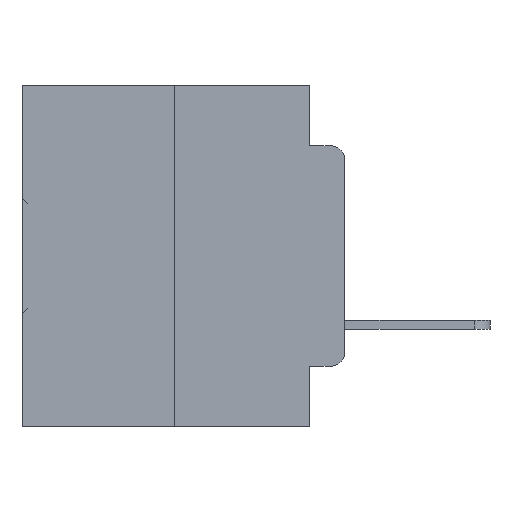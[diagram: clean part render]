
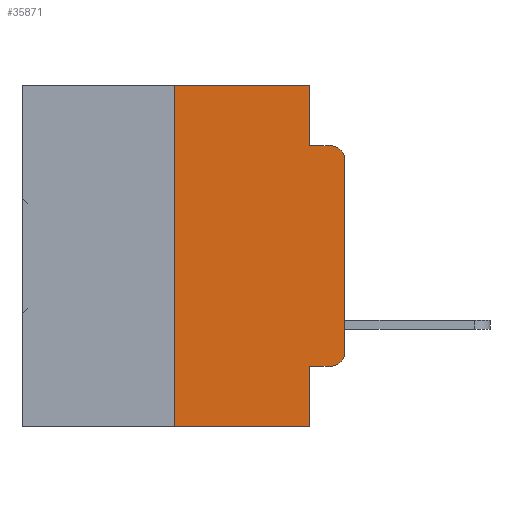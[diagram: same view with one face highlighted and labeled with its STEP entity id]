
A CAD part, left-side view. The second image highlights one B-rep face of the part: STEP entity #35871.
In plain terms, the highlighted planar face has unit normal (-1, 0, 0).
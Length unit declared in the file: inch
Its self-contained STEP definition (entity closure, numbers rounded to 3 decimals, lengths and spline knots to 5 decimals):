
#380 = EDGE_CURVE ( 'NONE', #27012, #5981, #12799, .T. ) ;
#2295 = EDGE_CURVE ( 'NONE', #11353, #27012, #8159, .T. ) ;
#2344 = EDGE_CURVE ( 'NONE', #18755, #28201, #34345, .T. ) ;
#4235 = EDGE_CURVE ( 'NONE', #11353, #32620, #6273, .T. ) ;
#4344 = VERTEX_POINT ( 'NONE', #6306 ) ;
#4665 = VECTOR ( 'NONE', #10213, 39.37008 ) ;
#4811 = VERTEX_POINT ( 'NONE', #8684 ) ;
#4935 = ORIENTED_EDGE ( 'NONE', *, *, #17738, .F. ) ;
#5347 = DIRECTION ( 'NONE',  ( 0., 0., 1. ) ) ;
#5734 = VERTEX_POINT ( 'NONE', #20676 ) ;
#5981 = VERTEX_POINT ( 'NONE', #10406 ) ;
#6125 = DIRECTION ( 'NONE',  ( 0., 0., -1. ) ) ;
#6170 = EDGE_CURVE ( 'NONE', #5734, #18755, #30769, .T. ) ;
#6264 = CARTESIAN_POINT ( 'NONE',  ( 0., 0.051, -0.5 ) ) ;
#6273 = LINE ( 'NONE', #8712, #20634 ) ;
#6306 = CARTESIAN_POINT ( 'NONE',  ( 0., 0.051, -0.0885 ) ) ;
#6311 = EDGE_LOOP ( 'NONE', ( #21344, #27413, #25255, #4935, #19779, #27445, #12371, #16758, #21984, #7515 ) ) ;
#7210 = DIRECTION ( 'NONE',  ( -1., 0., 0. ) ) ;
#7326 = CARTESIAN_POINT ( 'NONE',  ( 0., 0.051, -0.0885 ) ) ;
#7515 = ORIENTED_EDGE ( 'NONE', *, *, #380, .T. ) ;
#8159 = LINE ( 'NONE', #27965, #13971 ) ;
#8195 = LINE ( 'NONE', #25158, #14007 ) ;
#8247 = CARTESIAN_POINT ( 'NONE',  ( 0., 0.25, 0. ) ) ;
#8450 = AXIS2_PLACEMENT_3D ( 'NONE', #24183, #7210, #26970 ) ;
#8602 = PLANE ( 'NONE',  #15522 ) ;
#8684 = CARTESIAN_POINT ( 'NONE',  ( 0., 0.02, -0.0885 ) ) ;
#8712 = CARTESIAN_POINT ( 'NONE',  ( 0., 0.051, 0. ) ) ;
#10178 = CARTESIAN_POINT ( 'NONE',  ( 0., 0.051, -0.4115 ) ) ;
#10213 = DIRECTION ( 'NONE',  ( 0., -1., 0. ) ) ;
#10406 = CARTESIAN_POINT ( 'NONE',  ( 0., 0., -0.3915 ) ) ;
#10719 = CARTESIAN_POINT ( 'NONE',  ( 0., 0.473, -0.5 ) ) ;
#11011 = CARTESIAN_POINT ( 'NONE',  ( 0., 0.051, 0. ) ) ;
#11353 = VERTEX_POINT ( 'NONE', #10178 ) ;
#11428 = LINE ( 'NONE', #11011, #25590 ) ;
#12371 = ORIENTED_EDGE ( 'NONE', *, *, #26844, .T. ) ;
#12799 = CIRCLE ( 'NONE', #13096, 0.02 ) ;
#13096 = AXIS2_PLACEMENT_3D ( 'NONE', #14127, #33549, #17056 ) ;
#13809 = DIRECTION ( 'NONE',  ( 0., 0., 1. ) ) ;
#13971 = VECTOR ( 'NONE', #28083, 39.37008 ) ;
#14007 = VECTOR ( 'NONE', #13809, 39.37008 ) ;
#14127 = CARTESIAN_POINT ( 'NONE',  ( 0., 0.02, -0.3915 ) ) ;
#15522 = AXIS2_PLACEMENT_3D ( 'NONE', #33758, #17275, #6125 ) ;
#15587 = VERTEX_POINT ( 'NONE', #25623 ) ;
#16025 = VECTOR ( 'NONE', #5347, 39.37008 ) ;
#16758 = ORIENTED_EDGE ( 'NONE', *, *, #4235, .F. ) ;
#17056 = DIRECTION ( 'NONE',  ( 0., 0., -1. ) ) ;
#17275 = DIRECTION ( 'NONE',  ( 1., 0., 0. ) ) ;
#17738 = EDGE_CURVE ( 'NONE', #28201, #4344, #11428, .T. ) ;
#18173 = CIRCLE ( 'NONE', #8450, 0.02 ) ;
#18755 = VERTEX_POINT ( 'NONE', #28562 ) ;
#19598 = VECTOR ( 'NONE', #30289, 39.37008 ) ;
#19684 = EDGE_CURVE ( 'NONE', #4344, #4811, #19969, .T. ) ;
#19779 = ORIENTED_EDGE ( 'NONE', *, *, #2344, .F. ) ;
#19847 = VECTOR ( 'NONE', #26051, 39.37008 ) ;
#19969 = LINE ( 'NONE', #7326, #4665 ) ;
#20634 = VECTOR ( 'NONE', #28409, 39.37008 ) ;
#20676 = CARTESIAN_POINT ( 'NONE',  ( 0., 0.25, -0.5 ) ) ;
#21344 = ORIENTED_EDGE ( 'NONE', *, *, #30696, .T. ) ;
#21545 = EDGE_CURVE ( 'NONE', #15587, #4811, #18173, .T. ) ;
#21984 = ORIENTED_EDGE ( 'NONE', *, *, #2295, .T. ) ;
#24183 = CARTESIAN_POINT ( 'NONE',  ( 0., 0.02, -0.1085 ) ) ;
#25158 = CARTESIAN_POINT ( 'NONE',  ( 0., 0., 0. ) ) ;
#25255 = ORIENTED_EDGE ( 'NONE', *, *, #19684, .F. ) ;
#25590 = VECTOR ( 'NONE', #33322, 39.37008 ) ;
#25623 = CARTESIAN_POINT ( 'NONE',  ( 0., 0., -0.1085 ) ) ;
#26051 = DIRECTION ( 'NONE',  ( 0., -1., 0. ) ) ;
#26173 = CARTESIAN_POINT ( 'NONE',  ( 0., 0.051, 0. ) ) ;
#26844 = EDGE_CURVE ( 'NONE', #5734, #32620, #34123, .T. ) ;
#26970 = DIRECTION ( 'NONE',  ( 0., 0., -1. ) ) ;
#27012 = VERTEX_POINT ( 'NONE', #34202 ) ;
#27413 = ORIENTED_EDGE ( 'NONE', *, *, #21545, .T. ) ;
#27445 = ORIENTED_EDGE ( 'NONE', *, *, #6170, .F. ) ;
#27965 = CARTESIAN_POINT ( 'NONE',  ( 0., 0.051, -0.4115 ) ) ;
#28083 = DIRECTION ( 'NONE',  ( 0., -1., 0. ) ) ;
#28201 = VERTEX_POINT ( 'NONE', #26173 ) ;
#28409 = DIRECTION ( 'NONE',  ( 0., 0., -1. ) ) ;
#28562 = CARTESIAN_POINT ( 'NONE',  ( 0., 0.25, 0. ) ) ;
#28573 = FACE_OUTER_BOUND ( 'NONE', #6311, .T. ) ;
#28670 = CARTESIAN_POINT ( 'NONE',  ( 0., 0.473, 0. ) ) ;
#30289 = DIRECTION ( 'NONE',  ( 0., -1., 0. ) ) ;
#30696 = EDGE_CURVE ( 'NONE', #5981, #15587, #8195, .T. ) ;
#30769 = LINE ( 'NONE', #8247, #16025 ) ;
#32620 = VERTEX_POINT ( 'NONE', #6264 ) ;
#33322 = DIRECTION ( 'NONE',  ( 0., 0., -1. ) ) ;
#33549 = DIRECTION ( 'NONE',  ( -1., 0., 0. ) ) ;
#33758 = CARTESIAN_POINT ( 'NONE',  ( 0., 0.473, 0. ) ) ;
#34123 = LINE ( 'NONE', #10719, #19598 ) ;
#34202 = CARTESIAN_POINT ( 'NONE',  ( 0., 0.02, -0.4115 ) ) ;
#34345 = LINE ( 'NONE', #28670, #19847 ) ;
#35871 = ADVANCED_FACE ( 'NONE', ( #28573 ), #8602, .F. ) ;
